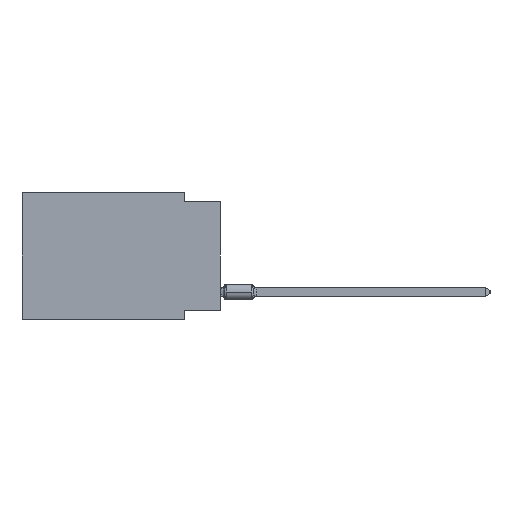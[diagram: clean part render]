
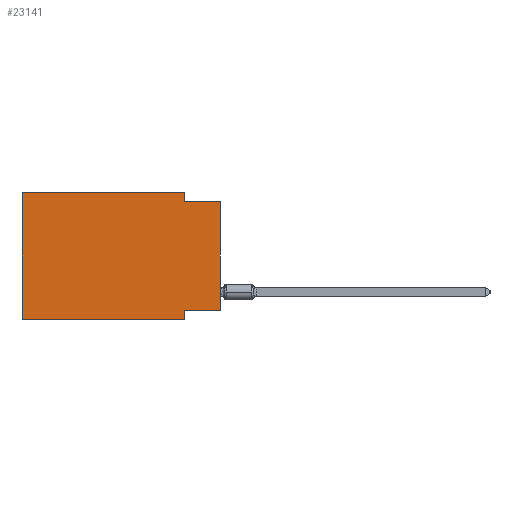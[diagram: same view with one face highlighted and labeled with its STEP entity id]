
A CAD part, left-side view. The second image highlights one B-rep face of the part: STEP entity #23141.
In plain terms, the highlighted planar face has unit normal (-1, 0, 0).
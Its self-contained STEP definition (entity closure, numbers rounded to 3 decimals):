
#71 = VERTEX_POINT ( 'NONE', #324 ) ;
#324 = CARTESIAN_POINT ( 'NONE',  ( 0., 0., -0.635 ) ) ;
#362 = EDGE_CURVE ( 'NONE', #12628, #7394, #17449, .T. ) ;
#464 = ORIENTED_EDGE ( 'NONE', *, *, #22119, .T. ) ;
#1214 = LINE ( 'NONE', #13618, #21969 ) ;
#1454 = VECTOR ( 'NONE', #1541, 1000. ) ;
#1541 = DIRECTION ( 'NONE',  ( 0., 0., 1. ) ) ;
#2107 = DIRECTION ( 'NONE',  ( 1., 0., 0. ) ) ;
#2447 = PLANE ( 'NONE',  #20496 ) ;
#2738 = VERTEX_POINT ( 'NONE', #6670 ) ;
#2776 = ORIENTED_EDGE ( 'NONE', *, *, #12165, .F. ) ;
#3057 = CARTESIAN_POINT ( 'NONE',  ( 0., 0., -0.635 ) ) ;
#3228 = DIRECTION ( 'NONE',  ( 0., -1., 0. ) ) ;
#3710 = ORIENTED_EDGE ( 'NONE', *, *, #13597, .F. ) ;
#3768 = LINE ( 'NONE', #32253, #17949 ) ;
#4206 = DIRECTION ( 'NONE',  ( 0., -1., 0. ) ) ;
#5760 = CARTESIAN_POINT ( 'NONE',  ( 0., 2.54, -8.255 ) ) ;
#5813 = DIRECTION ( 'NONE',  ( 0., 0., -1. ) ) ;
#6670 = CARTESIAN_POINT ( 'NONE',  ( 0., 13.97, -8.89 ) ) ;
#6811 = DIRECTION ( 'NONE',  ( 0., 0., -1. ) ) ;
#6952 = ORIENTED_EDGE ( 'NONE', *, *, #30207, .F. ) ;
#7048 = DIRECTION ( 'NONE',  ( 0., 0., -1. ) ) ;
#7394 = VERTEX_POINT ( 'NONE', #29700 ) ;
#8540 = EDGE_CURVE ( 'NONE', #2738, #12628, #24982, .T. ) ;
#8588 = CARTESIAN_POINT ( 'NONE',  ( 0., 2.54, -8.89 ) ) ;
#9035 = ORIENTED_EDGE ( 'NONE', *, *, #362, .F. ) ;
#9598 = FACE_OUTER_BOUND ( 'NONE', #28091, .T. ) ;
#9742 = CARTESIAN_POINT ( 'NONE',  ( 0., 13.97, -8.89 ) ) ;
#11152 = CARTESIAN_POINT ( 'NONE',  ( 0., 13.97, 0. ) ) ;
#11366 = VECTOR ( 'NONE', #3228, 1000. ) ;
#11904 = EDGE_CURVE ( 'NONE', #7394, #30841, #1214, .T. ) ;
#12165 = EDGE_CURVE ( 'NONE', #30841, #71, #23274, .T. ) ;
#12628 = VERTEX_POINT ( 'NONE', #11152 ) ;
#13289 = VECTOR ( 'NONE', #20094, 1000. ) ;
#13597 = EDGE_CURVE ( 'NONE', #18814, #26550, #3768, .T. ) ;
#13618 = CARTESIAN_POINT ( 'NONE',  ( 0., 2.54, 0. ) ) ;
#13881 = ORIENTED_EDGE ( 'NONE', *, *, #30961, .T. ) ;
#15067 = CARTESIAN_POINT ( 'NONE',  ( 0., 13.97, 0. ) ) ;
#15124 = CARTESIAN_POINT ( 'NONE',  ( 0., 2.54, -8.89 ) ) ;
#15141 = CARTESIAN_POINT ( 'NONE',  ( 0., 13.97, 0. ) ) ;
#15251 = VECTOR ( 'NONE', #17688, 1000. ) ;
#16840 = DIRECTION ( 'NONE',  ( 0., 1., 0. ) ) ;
#17038 = CARTESIAN_POINT ( 'NONE',  ( 0., 2.54, -0.635 ) ) ;
#17449 = LINE ( 'NONE', #15067, #26819 ) ;
#17688 = DIRECTION ( 'NONE',  ( 0., 0., 1. ) ) ;
#17949 = VECTOR ( 'NONE', #16840, 1000. ) ;
#18814 = VERTEX_POINT ( 'NONE', #24699 ) ;
#19953 = CARTESIAN_POINT ( 'NONE',  ( 0., 13.97, 0. ) ) ;
#20094 = DIRECTION ( 'NONE',  ( 0., -1., 0. ) ) ;
#20429 = LINE ( 'NONE', #9742, #13289 ) ;
#20496 = AXIS2_PLACEMENT_3D ( 'NONE', #19953, #2107, #7048 ) ;
#21013 = ORIENTED_EDGE ( 'NONE', *, *, #8540, .F. ) ;
#21223 = VERTEX_POINT ( 'NONE', #8588 ) ;
#21969 = VECTOR ( 'NONE', #5813, 1000. ) ;
#22119 = EDGE_CURVE ( 'NONE', #18814, #71, #26830, .T. ) ;
#23141 = ADVANCED_FACE ( 'NONE', ( #9598 ), #2447, .F. ) ;
#23274 = LINE ( 'NONE', #3057, #11366 ) ;
#23629 = ORIENTED_EDGE ( 'NONE', *, *, #11904, .F. ) ;
#24699 = CARTESIAN_POINT ( 'NONE',  ( 0., 0., -8.255 ) ) ;
#24982 = LINE ( 'NONE', #15141, #15251 ) ;
#26550 = VERTEX_POINT ( 'NONE', #5760 ) ;
#26819 = VECTOR ( 'NONE', #4206, 1000. ) ;
#26830 = LINE ( 'NONE', #30048, #1454 ) ;
#28091 = EDGE_LOOP ( 'NONE', ( #464, #2776, #23629, #9035, #21013, #13881, #6952, #3710 ) ) ;
#29700 = CARTESIAN_POINT ( 'NONE',  ( 0., 2.54, 0. ) ) ;
#30048 = CARTESIAN_POINT ( 'NONE',  ( 0., 0., 0. ) ) ;
#30049 = LINE ( 'NONE', #15124, #30579 ) ;
#30207 = EDGE_CURVE ( 'NONE', #26550, #21223, #30049, .T. ) ;
#30579 = VECTOR ( 'NONE', #6811, 1000. ) ;
#30841 = VERTEX_POINT ( 'NONE', #17038 ) ;
#30961 = EDGE_CURVE ( 'NONE', #2738, #21223, #20429, .T. ) ;
#32253 = CARTESIAN_POINT ( 'NONE',  ( 0., 0., -8.255 ) ) ;
